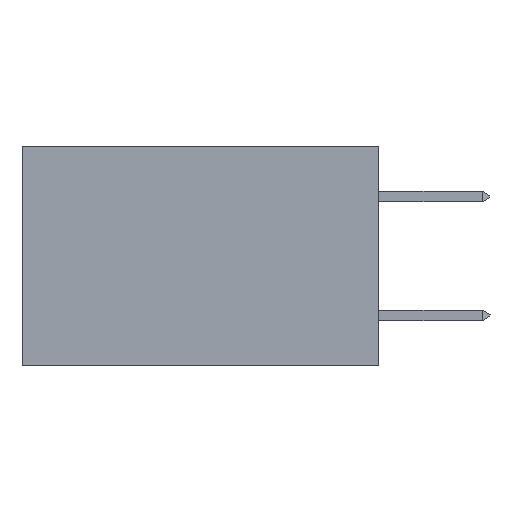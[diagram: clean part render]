
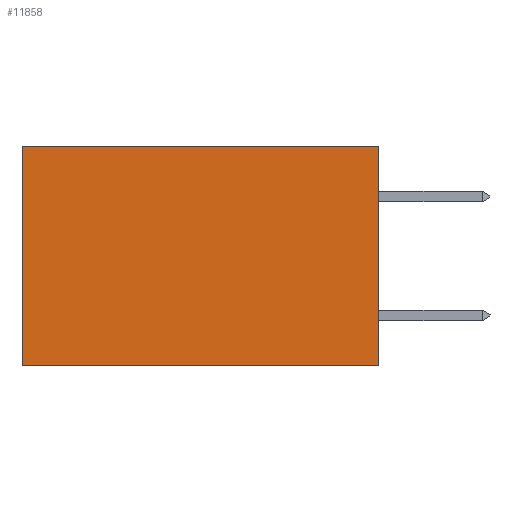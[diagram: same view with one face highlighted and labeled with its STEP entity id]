
A CAD part, left-side view. The second image highlights one B-rep face of the part: STEP entity #11858.
In plain terms, the highlighted planar face has unit normal (-1, 0, 0).
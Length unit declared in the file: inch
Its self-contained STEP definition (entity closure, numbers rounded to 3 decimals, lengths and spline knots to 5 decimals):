
#56 = ORIENTED_EDGE ( 'NONE', *, *, #6804, .F. ) ;
#200 = VERTEX_POINT ( 'NONE', #22968 ) ;
#598 = VECTOR ( 'NONE', #25080, 39.37008 ) ;
#1594 = VECTOR ( 'NONE', #19331, 39.37008 ) ;
#3056 = LINE ( 'NONE', #4007, #6740 ) ;
#4007 = CARTESIAN_POINT ( 'NONE',  ( 0.298, 0., -0.37 ) ) ;
#4281 = EDGE_CURVE ( 'NONE', #200, #18704, #13219, .T. ) ;
#5528 = ORIENTED_EDGE ( 'NONE', *, *, #23016, .T. ) ;
#6740 = VECTOR ( 'NONE', #7684, 39.37008 ) ;
#6804 = EDGE_CURVE ( 'NONE', #18704, #16492, #3056, .T. ) ;
#7192 = EDGE_LOOP ( 'NONE', ( #5528, #56, #20301, #10493 ) ) ;
#7684 = DIRECTION ( 'NONE',  ( 0., 1., 0. ) ) ;
#7783 = CARTESIAN_POINT ( 'NONE',  ( 0.298, 0., -0.37 ) ) ;
#9068 = LINE ( 'NONE', #21776, #23433 ) ;
#10493 = ORIENTED_EDGE ( 'NONE', *, *, #24021, .T. ) ;
#11414 = DIRECTION ( 'NONE',  ( 1., 0., 0. ) ) ;
#11482 = CARTESIAN_POINT ( 'NONE',  ( 0.298, 0.6, 0. ) ) ;
#11723 = AXIS2_PLACEMENT_3D ( 'NONE', #20370, #11414, #15102 ) ;
#11858 = ADVANCED_FACE ( 'NONE', ( #18717 ), #16259, .F. ) ;
#13219 = LINE ( 'NONE', #23011, #1594 ) ;
#14339 = CARTESIAN_POINT ( 'NONE',  ( 0.298, 0.6, -0.37 ) ) ;
#15102 = DIRECTION ( 'NONE',  ( 0., 0., -1. ) ) ;
#16259 = PLANE ( 'NONE',  #11723 ) ;
#16429 = CARTESIAN_POINT ( 'NONE',  ( 0.298, 0.6, 0. ) ) ;
#16492 = VERTEX_POINT ( 'NONE', #14339 ) ;
#18037 = DIRECTION ( 'NONE',  ( 0., 1., 0. ) ) ;
#18704 = VERTEX_POINT ( 'NONE', #7783 ) ;
#18717 = FACE_OUTER_BOUND ( 'NONE', #7192, .T. ) ;
#19331 = DIRECTION ( 'NONE',  ( 0., 0., -1. ) ) ;
#20301 = ORIENTED_EDGE ( 'NONE', *, *, #4281, .F. ) ;
#20370 = CARTESIAN_POINT ( 'NONE',  ( 0.298, 0., 0. ) ) ;
#21776 = CARTESIAN_POINT ( 'NONE',  ( 0.298, 0., 0. ) ) ;
#21984 = LINE ( 'NONE', #11482, #598 ) ;
#22968 = CARTESIAN_POINT ( 'NONE',  ( 0.298, 0., 0. ) ) ;
#23011 = CARTESIAN_POINT ( 'NONE',  ( 0.298, 0., 0. ) ) ;
#23016 = EDGE_CURVE ( 'NONE', #23566, #16492, #21984, .T. ) ;
#23433 = VECTOR ( 'NONE', #18037, 39.37008 ) ;
#23566 = VERTEX_POINT ( 'NONE', #16429 ) ;
#24021 = EDGE_CURVE ( 'NONE', #200, #23566, #9068, .T. ) ;
#25080 = DIRECTION ( 'NONE',  ( 0., 0., -1. ) ) ;
